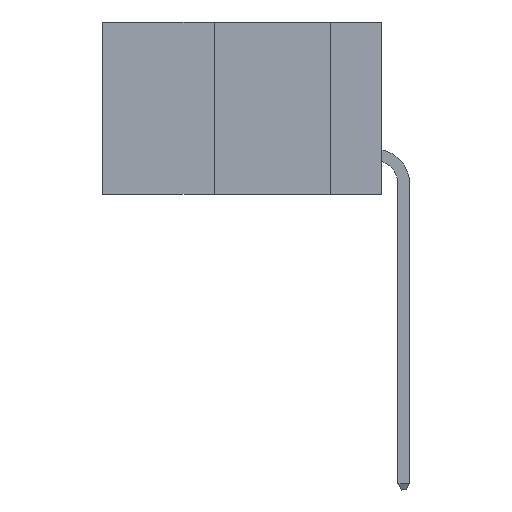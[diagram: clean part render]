
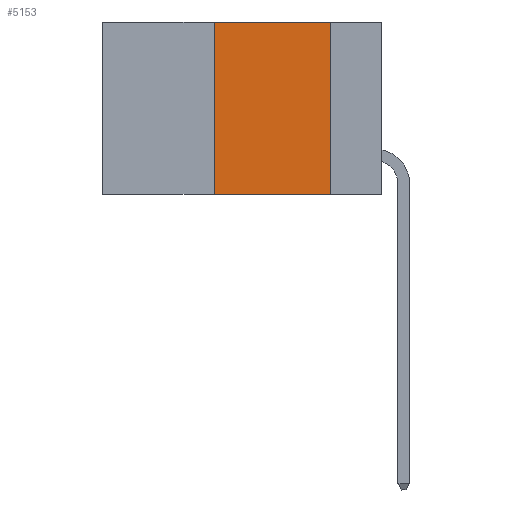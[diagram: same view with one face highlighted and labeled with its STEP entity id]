
A CAD part, left-side view. The second image highlights one B-rep face of the part: STEP entity #5153.
In plain terms, the highlighted planar face has unit normal (-1, 0, 0).
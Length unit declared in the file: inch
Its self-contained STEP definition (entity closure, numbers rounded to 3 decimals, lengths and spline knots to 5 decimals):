
#963 = CARTESIAN_POINT ( 'NONE',  ( 0., 0.36, 0. ) ) ;
#1026 = VERTEX_POINT ( 'NONE', #12114 ) ;
#1443 = LINE ( 'NONE', #11037, #7246 ) ;
#2428 = VERTEX_POINT ( 'NONE', #963 ) ;
#2742 = DIRECTION ( 'NONE',  ( 0., -1., 0. ) ) ;
#3530 = VERTEX_POINT ( 'NONE', #11479 ) ;
#3862 = EDGE_CURVE ( 'NONE', #2428, #1026, #13075, .T. ) ;
#4137 = EDGE_CURVE ( 'NONE', #13760, #2428, #6995, .T. ) ;
#4168 = VECTOR ( 'NONE', #9545, 39.37008 ) ;
#4808 = AXIS2_PLACEMENT_3D ( 'NONE', #11259, #4957, #12306 ) ;
#4892 = CARTESIAN_POINT ( 'NONE',  ( 0., 0.6, 0. ) ) ;
#4957 = DIRECTION ( 'NONE',  ( 1., 0., 0. ) ) ;
#5153 = ADVANCED_FACE ( 'NONE', ( #12881 ), #13317, .F. ) ;
#5280 = CARTESIAN_POINT ( 'NONE',  ( 0., 0.36, -0.37 ) ) ;
#5316 = EDGE_CURVE ( 'NONE', #13760, #3530, #11238, .T. ) ;
#5817 = DIRECTION ( 'NONE',  ( 0., 0., -1. ) ) ;
#6995 = LINE ( 'NONE', #7479, #4168 ) ;
#7246 = VECTOR ( 'NONE', #5817, 39.37008 ) ;
#7479 = CARTESIAN_POINT ( 'NONE',  ( 0., 0.36, 0. ) ) ;
#7498 = VECTOR ( 'NONE', #2742, 39.37008 ) ;
#7934 = EDGE_CURVE ( 'NONE', #1026, #3530, #1443, .T. ) ;
#8348 = CARTESIAN_POINT ( 'NONE',  ( 0., 0.6, -0.37 ) ) ;
#9545 = DIRECTION ( 'NONE',  ( 0., 0., 1. ) ) ;
#10071 = EDGE_LOOP ( 'NONE', ( #12516, #12299, #12680, #12790 ) ) ;
#11037 = CARTESIAN_POINT ( 'NONE',  ( 0., 0.11, 0. ) ) ;
#11238 = LINE ( 'NONE', #8348, #11566 ) ;
#11259 = CARTESIAN_POINT ( 'NONE',  ( 0., 0.6, 0. ) ) ;
#11479 = CARTESIAN_POINT ( 'NONE',  ( 0., 0.11, -0.37 ) ) ;
#11566 = VECTOR ( 'NONE', #12533, 39.37008 ) ;
#12114 = CARTESIAN_POINT ( 'NONE',  ( 0., 0.11, 0. ) ) ;
#12299 = ORIENTED_EDGE ( 'NONE', *, *, #3862, .F. ) ;
#12306 = DIRECTION ( 'NONE',  ( 0., 0., -1. ) ) ;
#12516 = ORIENTED_EDGE ( 'NONE', *, *, #7934, .F. ) ;
#12533 = DIRECTION ( 'NONE',  ( 0., -1., 0. ) ) ;
#12680 = ORIENTED_EDGE ( 'NONE', *, *, #4137, .F. ) ;
#12790 = ORIENTED_EDGE ( 'NONE', *, *, #5316, .T. ) ;
#12881 = FACE_OUTER_BOUND ( 'NONE', #10071, .T. ) ;
#13075 = LINE ( 'NONE', #4892, #7498 ) ;
#13317 = PLANE ( 'NONE',  #4808 ) ;
#13760 = VERTEX_POINT ( 'NONE', #5280 ) ;
